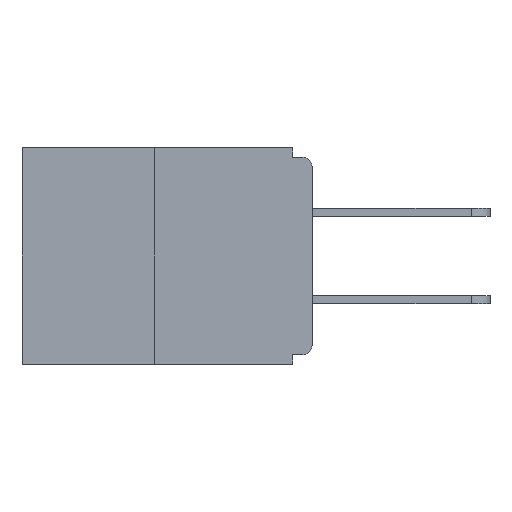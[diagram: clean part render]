
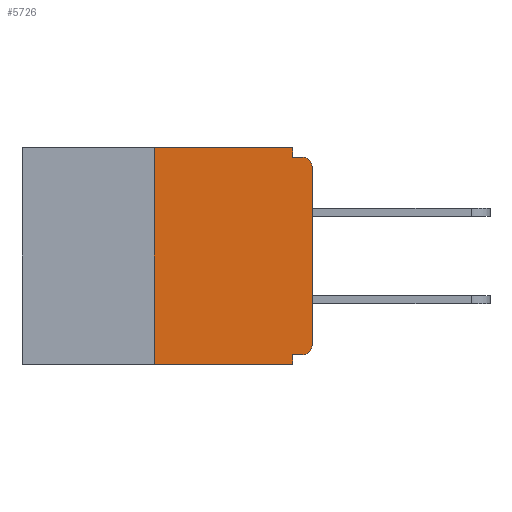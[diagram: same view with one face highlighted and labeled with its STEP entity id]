
A CAD part, left-side view. The second image highlights one B-rep face of the part: STEP entity #5726.
In plain terms, the highlighted planar face has unit normal (-1, 0, 0).
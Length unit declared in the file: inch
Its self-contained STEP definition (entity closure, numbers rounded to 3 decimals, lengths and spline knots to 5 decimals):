
#252 = LINE ( 'NONE', #16006, #11082 ) ;
#371 = FACE_OUTER_BOUND ( 'NONE', #16175, .T. ) ;
#624 = ORIENTED_EDGE ( 'NONE', *, *, #1358, .T. ) ;
#798 = CARTESIAN_POINT ( 'NONE',  ( 0., 0.015, -0.03 ) ) ;
#1236 = ORIENTED_EDGE ( 'NONE', *, *, #11277, .T. ) ;
#1358 = EDGE_CURVE ( 'NONE', #4144, #3963, #21998, .T. ) ;
#1605 = VECTOR ( 'NONE', #19772, 39.37008 ) ;
#1841 = VERTEX_POINT ( 'NONE', #9572 ) ;
#2056 = VECTOR ( 'NONE', #9337, 39.37008 ) ;
#2714 = LINE ( 'NONE', #16300, #1605 ) ;
#2781 = VECTOR ( 'NONE', #21563, 39.37008 ) ;
#3058 = DIRECTION ( 'NONE',  ( 1., 0., 0. ) ) ;
#3204 = CARTESIAN_POINT ( 'NONE',  ( 0., 0.46, 0. ) ) ;
#3855 = DIRECTION ( 'NONE',  ( 0., 0., 1. ) ) ;
#3963 = VERTEX_POINT ( 'NONE', #21962 ) ;
#4144 = VERTEX_POINT ( 'NONE', #8916 ) ;
#4223 = CARTESIAN_POINT ( 'NONE',  ( 0., 0.46, 0. ) ) ;
#4335 = EDGE_CURVE ( 'NONE', #20519, #19683, #11275, .T. ) ;
#4384 = DIRECTION ( 'NONE',  ( 0., 0., -1. ) ) ;
#4391 = AXIS2_PLACEMENT_3D ( 'NONE', #3204, #3058, #22061 ) ;
#4979 = CARTESIAN_POINT ( 'NONE',  ( 0., 0.25, -0.343 ) ) ;
#4991 = VERTEX_POINT ( 'NONE', #6507 ) ;
#5369 = VECTOR ( 'NONE', #7495, 39.37008 ) ;
#5541 = CARTESIAN_POINT ( 'NONE',  ( 0., 0.25, 0. ) ) ;
#5713 = LINE ( 'NONE', #6530, #11931 ) ;
#5726 = ADVANCED_FACE ( 'NONE', ( #371 ), #18786, .F. ) ;
#5975 = ORIENTED_EDGE ( 'NONE', *, *, #17641, .F. ) ;
#6175 = CARTESIAN_POINT ( 'NONE',  ( 0., 0.46, -0.343 ) ) ;
#6507 = CARTESIAN_POINT ( 'NONE',  ( 0., 0.015, -0.015 ) ) ;
#6530 = CARTESIAN_POINT ( 'NONE',  ( 0., 0., 0. ) ) ;
#6811 = ORIENTED_EDGE ( 'NONE', *, *, #11295, .F. ) ;
#6899 = EDGE_CURVE ( 'NONE', #13674, #9254, #15518, .T. ) ;
#7495 = DIRECTION ( 'NONE',  ( 0., -1., 0. ) ) ;
#7640 = ORIENTED_EDGE ( 'NONE', *, *, #9363, .F. ) ;
#7672 = DIRECTION ( 'NONE',  ( 0., 0., 1. ) ) ;
#7720 = ORIENTED_EDGE ( 'NONE', *, *, #18331, .F. ) ;
#7824 = ORIENTED_EDGE ( 'NONE', *, *, #20309, .F. ) ;
#8212 = VECTOR ( 'NONE', #4384, 39.37008 ) ;
#8308 = LINE ( 'NONE', #11050, #5369 ) ;
#8347 = ORIENTED_EDGE ( 'NONE', *, *, #6899, .F. ) ;
#8916 = CARTESIAN_POINT ( 'NONE',  ( 0., 0.015, -0.328 ) ) ;
#9254 = VERTEX_POINT ( 'NONE', #21901 ) ;
#9337 = DIRECTION ( 'NONE',  ( 0., -1., 0. ) ) ;
#9363 = EDGE_CURVE ( 'NONE', #20519, #13674, #17806, .T. ) ;
#9572 = CARTESIAN_POINT ( 'NONE',  ( 0., 0.031, -0.328 ) ) ;
#9574 = DIRECTION ( 'NONE',  ( -1., 0., 0. ) ) ;
#9949 = EDGE_CURVE ( 'NONE', #19424, #4991, #16063, .T. ) ;
#11050 = CARTESIAN_POINT ( 'NONE',  ( 0., 0., -0.015 ) ) ;
#11082 = VECTOR ( 'NONE', #12464, 39.37008 ) ;
#11208 = LINE ( 'NONE', #11332, #8212 ) ;
#11275 = LINE ( 'NONE', #6175, #2056 ) ;
#11277 = EDGE_CURVE ( 'NONE', #3963, #19424, #5713, .T. ) ;
#11295 = EDGE_CURVE ( 'NONE', #4144, #1841, #2714, .T. ) ;
#11332 = CARTESIAN_POINT ( 'NONE',  ( 0., 0.031, -0.343 ) ) ;
#11931 = VECTOR ( 'NONE', #7672, 39.37008 ) ;
#12464 = DIRECTION ( 'NONE',  ( 0., 0., -1. ) ) ;
#12848 = DIRECTION ( 'NONE',  ( -1., 0., 0. ) ) ;
#12987 = DIRECTION ( 'NONE',  ( 0., 0., -1. ) ) ;
#13197 = VECTOR ( 'NONE', #3855, 39.37008 ) ;
#13674 = VERTEX_POINT ( 'NONE', #20577 ) ;
#15518 = LINE ( 'NONE', #4223, #2781 ) ;
#16006 = CARTESIAN_POINT ( 'NONE',  ( 0., 0.031, 0. ) ) ;
#16042 = CARTESIAN_POINT ( 'NONE',  ( 0., 0.031, -0.015 ) ) ;
#16063 = CIRCLE ( 'NONE', #20800, 0.015 ) ;
#16175 = EDGE_LOOP ( 'NONE', ( #8347, #7640, #21464, #7824, #6811, #624, #1236, #18719, #7720, #5975 ) ) ;
#16300 = CARTESIAN_POINT ( 'NONE',  ( 0., 0., -0.328 ) ) ;
#16429 = AXIS2_PLACEMENT_3D ( 'NONE', #20101, #9574, #12987 ) ;
#17641 = EDGE_CURVE ( 'NONE', #9254, #20214, #252, .T. ) ;
#17786 = CARTESIAN_POINT ( 'NONE',  ( 0., 0.031, -0.343 ) ) ;
#17806 = LINE ( 'NONE', #5541, #13197 ) ;
#18331 = EDGE_CURVE ( 'NONE', #20214, #4991, #8308, .T. ) ;
#18646 = CARTESIAN_POINT ( 'NONE',  ( 0., 0., -0.03 ) ) ;
#18719 = ORIENTED_EDGE ( 'NONE', *, *, #9949, .T. ) ;
#18786 = PLANE ( 'NONE',  #4391 ) ;
#19424 = VERTEX_POINT ( 'NONE', #18646 ) ;
#19652 = DIRECTION ( 'NONE',  ( 0., 0., -1. ) ) ;
#19683 = VERTEX_POINT ( 'NONE', #17786 ) ;
#19772 = DIRECTION ( 'NONE',  ( 0., 1., 0. ) ) ;
#20101 = CARTESIAN_POINT ( 'NONE',  ( 0., 0.015, -0.313 ) ) ;
#20214 = VERTEX_POINT ( 'NONE', #16042 ) ;
#20309 = EDGE_CURVE ( 'NONE', #1841, #19683, #11208, .T. ) ;
#20519 = VERTEX_POINT ( 'NONE', #4979 ) ;
#20577 = CARTESIAN_POINT ( 'NONE',  ( 0., 0.25, 0. ) ) ;
#20800 = AXIS2_PLACEMENT_3D ( 'NONE', #798, #12848, #19652 ) ;
#21464 = ORIENTED_EDGE ( 'NONE', *, *, #4335, .T. ) ;
#21563 = DIRECTION ( 'NONE',  ( 0., -1., 0. ) ) ;
#21901 = CARTESIAN_POINT ( 'NONE',  ( 0., 0.031, 0. ) ) ;
#21962 = CARTESIAN_POINT ( 'NONE',  ( 0., 0., -0.313 ) ) ;
#21998 = CIRCLE ( 'NONE', #16429, 0.015 ) ;
#22061 = DIRECTION ( 'NONE',  ( 0., 0., -1. ) ) ;
